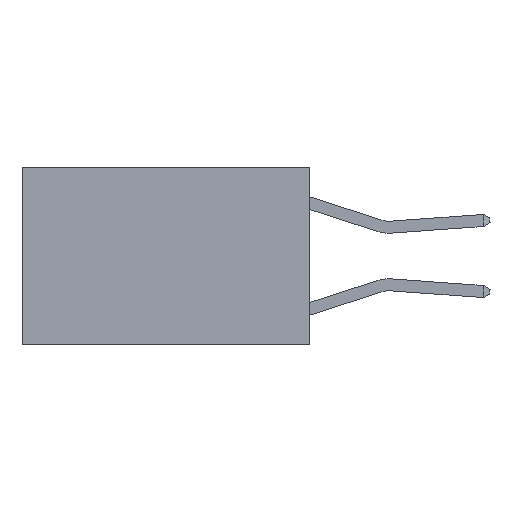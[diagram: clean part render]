
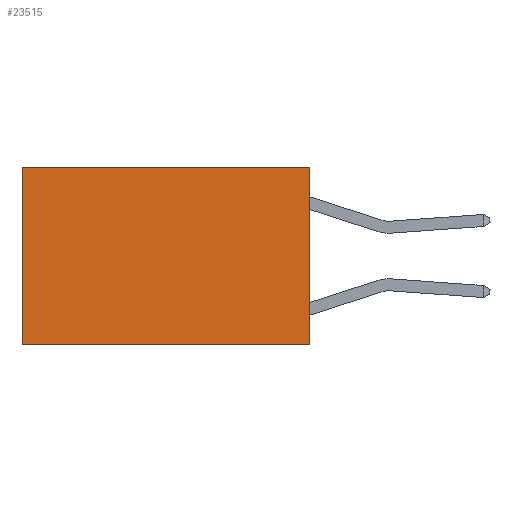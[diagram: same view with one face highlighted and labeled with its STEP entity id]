
A CAD part, left-side view. The second image highlights one B-rep face of the part: STEP entity #23515.
In plain terms, the highlighted planar face has unit normal (-1, 0, 0).
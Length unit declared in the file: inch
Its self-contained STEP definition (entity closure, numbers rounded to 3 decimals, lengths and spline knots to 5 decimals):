
#335 = CARTESIAN_POINT ( 'NONE',  ( 0.2625, 0.6, -0.37 ) ) ;
#884 = EDGE_CURVE ( 'NONE', #8779, #13279, #12317, .T. ) ;
#1464 = CARTESIAN_POINT ( 'NONE',  ( 0.2625, 0.6, 0. ) ) ;
#2096 = ORIENTED_EDGE ( 'NONE', *, *, #9472, .F. ) ;
#2683 = LINE ( 'NONE', #16009, #14235 ) ;
#2776 = ORIENTED_EDGE ( 'NONE', *, *, #884, .T. ) ;
#3711 = VECTOR ( 'NONE', #4779, 39.37008 ) ;
#4779 = DIRECTION ( 'NONE',  ( 0., 0., -1. ) ) ;
#6778 = LINE ( 'NONE', #13504, #3711 ) ;
#6992 = DIRECTION ( 'NONE',  ( 0., 1., 0. ) ) ;
#7011 = CARTESIAN_POINT ( 'NONE',  ( 0.2625, 0., 0. ) ) ;
#8586 = DIRECTION ( 'NONE',  ( 0., 0., -1. ) ) ;
#8611 = CARTESIAN_POINT ( 'NONE',  ( 0.2625, 0., 0. ) ) ;
#8779 = VERTEX_POINT ( 'NONE', #27485 ) ;
#9088 = EDGE_CURVE ( 'NONE', #10513, #13279, #2683, .T. ) ;
#9472 = EDGE_CURVE ( 'NONE', #22852, #10513, #6778, .T. ) ;
#10513 = VERTEX_POINT ( 'NONE', #16598 ) ;
#11356 = VECTOR ( 'NONE', #22951, 39.37008 ) ;
#12317 = LINE ( 'NONE', #1464, #11356 ) ;
#12727 = DIRECTION ( 'NONE',  ( 1., 0., 0. ) ) ;
#13228 = VECTOR ( 'NONE', #19784, 39.37008 ) ;
#13279 = VERTEX_POINT ( 'NONE', #335 ) ;
#13504 = CARTESIAN_POINT ( 'NONE',  ( 0.2625, 0., 0. ) ) ;
#14235 = VECTOR ( 'NONE', #6992, 39.37008 ) ;
#14250 = ORIENTED_EDGE ( 'NONE', *, *, #9088, .F. ) ;
#15088 = LINE ( 'NONE', #8611, #13228 ) ;
#16009 = CARTESIAN_POINT ( 'NONE',  ( 0.2625, 0., -0.37 ) ) ;
#16598 = CARTESIAN_POINT ( 'NONE',  ( 0.2625, 0., -0.37 ) ) ;
#17487 = AXIS2_PLACEMENT_3D ( 'NONE', #23327, #12727, #8586 ) ;
#19285 = EDGE_LOOP ( 'NONE', ( #2776, #14250, #2096, #22837 ) ) ;
#19784 = DIRECTION ( 'NONE',  ( 0., 1., 0. ) ) ;
#20866 = EDGE_CURVE ( 'NONE', #22852, #8779, #15088, .T. ) ;
#21196 = FACE_OUTER_BOUND ( 'NONE', #19285, .T. ) ;
#22837 = ORIENTED_EDGE ( 'NONE', *, *, #20866, .T. ) ;
#22852 = VERTEX_POINT ( 'NONE', #7011 ) ;
#22951 = DIRECTION ( 'NONE',  ( 0., 0., -1. ) ) ;
#23327 = CARTESIAN_POINT ( 'NONE',  ( 0.2625, 0., 0. ) ) ;
#23515 = ADVANCED_FACE ( 'NONE', ( #21196 ), #25488, .F. ) ;
#25488 = PLANE ( 'NONE',  #17487 ) ;
#27485 = CARTESIAN_POINT ( 'NONE',  ( 0.2625, 0.6, 0. ) ) ;
